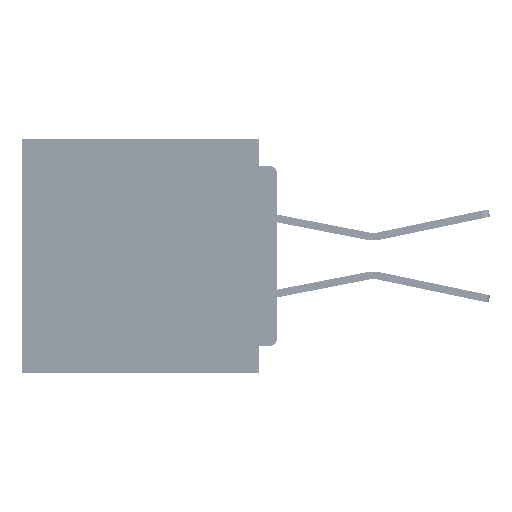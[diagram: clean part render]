
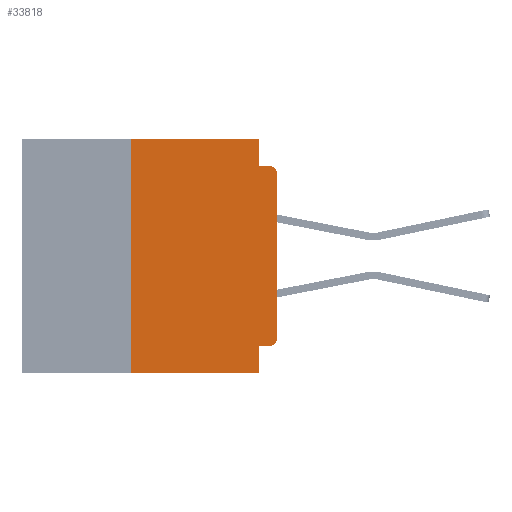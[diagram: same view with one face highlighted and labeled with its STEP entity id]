
A CAD part, left-side view. The second image highlights one B-rep face of the part: STEP entity #33818.
In plain terms, the highlighted planar face has unit normal (-1, 0, 0).
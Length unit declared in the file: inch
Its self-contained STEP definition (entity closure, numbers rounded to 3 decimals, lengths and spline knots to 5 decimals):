
#1133 = VECTOR ( 'NONE', #23986, 39.37008 ) ;
#2890 = VERTEX_POINT ( 'NONE', #57803 ) ;
#3666 = DIRECTION ( 'NONE',  ( 0., -1., 0. ) ) ;
#4232 = VERTEX_POINT ( 'NONE', #5369 ) ;
#4479 = DIRECTION ( 'NONE',  ( 0., -1., 0. ) ) ;
#5369 = CARTESIAN_POINT ( 'NONE',  ( 0., 0., -0.06 ) ) ;
#6314 = CARTESIAN_POINT ( 'NONE',  ( 0., 0.25, 0. ) ) ;
#6393 = EDGE_CURVE ( 'NONE', #21816, #41797, #54865, .T. ) ;
#6458 = CARTESIAN_POINT ( 'NONE',  ( 0., 0.031, -0.4 ) ) ;
#6535 = LINE ( 'NONE', #23785, #9745 ) ;
#7547 = VECTOR ( 'NONE', #3666, 39.37008 ) ;
#8510 = VECTOR ( 'NONE', #31624, 39.37008 ) ;
#9040 = ORIENTED_EDGE ( 'NONE', *, *, #28132, .F. ) ;
#9346 = CARTESIAN_POINT ( 'NONE',  ( 0., 0.031, -0.045 ) ) ;
#9623 = AXIS2_PLACEMENT_3D ( 'NONE', #11738, #47031, #16765 ) ;
#9745 = VECTOR ( 'NONE', #28904, 39.37008 ) ;
#9882 = EDGE_CURVE ( 'NONE', #4232, #11300, #38020, .T. ) ;
#10364 = VERTEX_POINT ( 'NONE', #9346 ) ;
#11300 = VERTEX_POINT ( 'NONE', #17217 ) ;
#11440 = CARTESIAN_POINT ( 'NONE',  ( 0., 0.031, 0. ) ) ;
#11738 = CARTESIAN_POINT ( 'NONE',  ( 0., 0.015, -0.34 ) ) ;
#12096 = VERTEX_POINT ( 'NONE', #58766 ) ;
#13918 = CARTESIAN_POINT ( 'NONE',  ( 0., 0.015, -0.06 ) ) ;
#14906 = EDGE_CURVE ( 'NONE', #2890, #4232, #49232, .T. ) ;
#16466 = CARTESIAN_POINT ( 'NONE',  ( 0., 0.015, -0.355 ) ) ;
#16763 = DIRECTION ( 'NONE',  ( 0., 0., 1. ) ) ;
#16765 = DIRECTION ( 'NONE',  ( 0., 0., -1. ) ) ;
#17217 = CARTESIAN_POINT ( 'NONE',  ( 0., 0.015, -0.045 ) ) ;
#17334 = DIRECTION ( 'NONE',  ( 1., 0., 0. ) ) ;
#17378 = FACE_OUTER_BOUND ( 'NONE', #18216, .T. ) ;
#17385 = CIRCLE ( 'NONE', #9623, 0.015 ) ;
#18216 = EDGE_LOOP ( 'NONE', ( #53810, #61545, #58642, #51841, #23547, #48672, #36382, #59591, #9040, #33782 ) ) ;
#18664 = CARTESIAN_POINT ( 'NONE',  ( 0., 0.437, -0.4 ) ) ;
#18756 = CARTESIAN_POINT ( 'NONE',  ( 0., 0.437, 0. ) ) ;
#18977 = DIRECTION ( 'NONE',  ( 0., 0., -1. ) ) ;
#21816 = VERTEX_POINT ( 'NONE', #57007 ) ;
#22641 = LINE ( 'NONE', #18756, #7547 ) ;
#22805 = VERTEX_POINT ( 'NONE', #6314 ) ;
#23547 = ORIENTED_EDGE ( 'NONE', *, *, #38263, .F. ) ;
#23597 = LINE ( 'NONE', #11440, #8510 ) ;
#23785 = CARTESIAN_POINT ( 'NONE',  ( 0., 0.25, -0.4 ) ) ;
#23986 = DIRECTION ( 'NONE',  ( 0., -1., 0. ) ) ;
#24676 = CARTESIAN_POINT ( 'NONE',  ( 0., 0., -0.045 ) ) ;
#25678 = VERTEX_POINT ( 'NONE', #46860 ) ;
#28120 = VECTOR ( 'NONE', #61570, 39.37008 ) ;
#28132 = EDGE_CURVE ( 'NONE', #61167, #21816, #52337, .T. ) ;
#28904 = DIRECTION ( 'NONE',  ( 0., 0., 1. ) ) ;
#31081 = EDGE_CURVE ( 'NONE', #10364, #11300, #33090, .T. ) ;
#31624 = DIRECTION ( 'NONE',  ( 0., 0., -1. ) ) ;
#33090 = LINE ( 'NONE', #24676, #58204 ) ;
#33445 = AXIS2_PLACEMENT_3D ( 'NONE', #13918, #49226, #18977 ) ;
#33782 = ORIENTED_EDGE ( 'NONE', *, *, #42491, .T. ) ;
#33818 = ADVANCED_FACE ( 'NONE', ( #17378 ), #47377, .F. ) ;
#36382 = ORIENTED_EDGE ( 'NONE', *, *, #65136, .T. ) ;
#38020 = CIRCLE ( 'NONE', #33445, 0.015 ) ;
#38263 = EDGE_CURVE ( 'NONE', #22805, #12096, #22641, .T. ) ;
#38995 = VECTOR ( 'NONE', #16763, 39.37008 ) ;
#41573 = CARTESIAN_POINT ( 'NONE',  ( 0., 0.031, -0.4 ) ) ;
#41797 = VERTEX_POINT ( 'NONE', #6458 ) ;
#42491 = EDGE_CURVE ( 'NONE', #61167, #2890, #17385, .T. ) ;
#44955 = EDGE_CURVE ( 'NONE', #12096, #10364, #23597, .T. ) ;
#46860 = CARTESIAN_POINT ( 'NONE',  ( 0., 0.25, -0.4 ) ) ;
#47027 = CARTESIAN_POINT ( 'NONE',  ( 0., 0., 0. ) ) ;
#47031 = DIRECTION ( 'NONE',  ( -1., 0., 0. ) ) ;
#47377 = PLANE ( 'NONE',  #64552 ) ;
#47582 = CARTESIAN_POINT ( 'NONE',  ( 0., 0.437, 0. ) ) ;
#48332 = EDGE_CURVE ( 'NONE', #25678, #22805, #6535, .T. ) ;
#48672 = ORIENTED_EDGE ( 'NONE', *, *, #48332, .F. ) ;
#49226 = DIRECTION ( 'NONE',  ( -1., 0., 0. ) ) ;
#49232 = LINE ( 'NONE', #47027, #38995 ) ;
#49396 = CARTESIAN_POINT ( 'NONE',  ( 0., 0., -0.355 ) ) ;
#51841 = ORIENTED_EDGE ( 'NONE', *, *, #44955, .F. ) ;
#52337 = LINE ( 'NONE', #49396, #64122 ) ;
#52620 = DIRECTION ( 'NONE',  ( 0., 0., -1. ) ) ;
#53810 = ORIENTED_EDGE ( 'NONE', *, *, #14906, .T. ) ;
#54861 = LINE ( 'NONE', #18664, #1133 ) ;
#54865 = LINE ( 'NONE', #41573, #28120 ) ;
#57007 = CARTESIAN_POINT ( 'NONE',  ( 0., 0.031, -0.355 ) ) ;
#57803 = CARTESIAN_POINT ( 'NONE',  ( 0., 0., -0.34 ) ) ;
#58204 = VECTOR ( 'NONE', #4479, 39.37008 ) ;
#58642 = ORIENTED_EDGE ( 'NONE', *, *, #31081, .F. ) ;
#58766 = CARTESIAN_POINT ( 'NONE',  ( 0., 0.031, 0. ) ) ;
#59591 = ORIENTED_EDGE ( 'NONE', *, *, #6393, .F. ) ;
#61167 = VERTEX_POINT ( 'NONE', #16466 ) ;
#61545 = ORIENTED_EDGE ( 'NONE', *, *, #9882, .T. ) ;
#61570 = DIRECTION ( 'NONE',  ( 0., 0., -1. ) ) ;
#64122 = VECTOR ( 'NONE', #64521, 39.37008 ) ;
#64521 = DIRECTION ( 'NONE',  ( 0., 1., 0. ) ) ;
#64552 = AXIS2_PLACEMENT_3D ( 'NONE', #47582, #17334, #52620 ) ;
#65136 = EDGE_CURVE ( 'NONE', #25678, #41797, #54861, .T. ) ;
